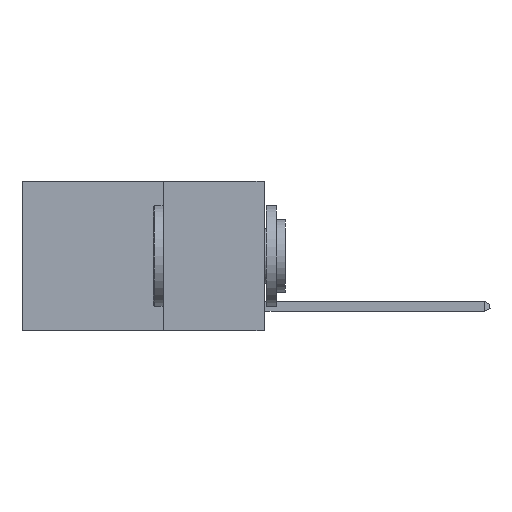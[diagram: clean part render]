
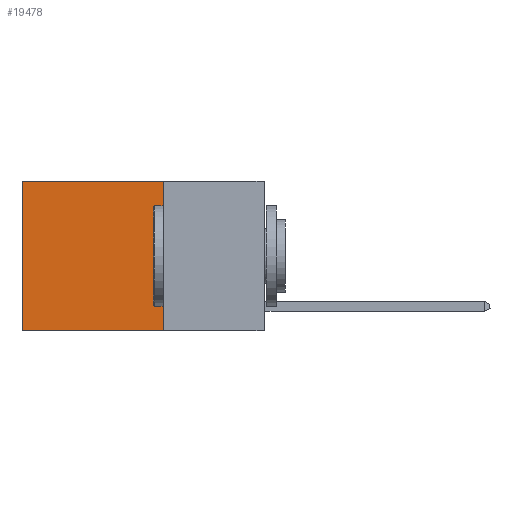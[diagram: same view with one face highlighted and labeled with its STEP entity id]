
A CAD part, left-side view. The second image highlights one B-rep face of the part: STEP entity #19478.
In plain terms, the highlighted planar face has unit normal (-1, 0, 0).
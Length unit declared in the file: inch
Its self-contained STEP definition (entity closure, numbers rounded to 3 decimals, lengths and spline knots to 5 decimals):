
#338 = CARTESIAN_POINT ( 'NONE',  ( 0.2625, 0.25, 0. ) ) ;
#354 = VECTOR ( 'NONE', #20214, 39.37008 ) ;
#499 = CARTESIAN_POINT ( 'NONE',  ( 0.2625, 0.25, 0. ) ) ;
#1576 = CARTESIAN_POINT ( 'NONE',  ( 0.2625, 0.25, -0.37 ) ) ;
#2954 = ORIENTED_EDGE ( 'NONE', *, *, #8389, .F. ) ;
#3614 = CARTESIAN_POINT ( 'NONE',  ( 0.2625, 0.6, 0. ) ) ;
#3741 = DIRECTION ( 'NONE',  ( 0., 0., -1. ) ) ;
#4375 = DIRECTION ( 'NONE',  ( 0., 0., -1. ) ) ;
#5207 = LINE ( 'NONE', #13923, #22955 ) ;
#5545 = CARTESIAN_POINT ( 'NONE',  ( 0.2625, 0.6, -0.37 ) ) ;
#5918 = FACE_OUTER_BOUND ( 'NONE', #6342, .T. ) ;
#6342 = EDGE_LOOP ( 'NONE', ( #15962, #17156, #2954, #9916 ) ) ;
#6417 = VECTOR ( 'NONE', #3741, 39.37008 ) ;
#7149 = LINE ( 'NONE', #338, #6417 ) ;
#7346 = VECTOR ( 'NONE', #10700, 39.37008 ) ;
#7847 = CARTESIAN_POINT ( 'NONE',  ( 0.2625, 0.6, 0. ) ) ;
#7977 = EDGE_CURVE ( 'NONE', #14332, #16102, #5207, .T. ) ;
#8014 = DIRECTION ( 'NONE',  ( 1., 0., 0. ) ) ;
#8389 = EDGE_CURVE ( 'NONE', #14332, #19967, #7149, .T. ) ;
#9604 = EDGE_CURVE ( 'NONE', #16102, #15600, #12453, .T. ) ;
#9916 = ORIENTED_EDGE ( 'NONE', *, *, #7977, .T. ) ;
#10388 = DIRECTION ( 'NONE',  ( 0., 1., 0. ) ) ;
#10700 = DIRECTION ( 'NONE',  ( 0., 0., -1. ) ) ;
#12453 = LINE ( 'NONE', #3614, #7346 ) ;
#13923 = CARTESIAN_POINT ( 'NONE',  ( 0.2625, 0.25, 0. ) ) ;
#14292 = AXIS2_PLACEMENT_3D ( 'NONE', #499, #8014, #4375 ) ;
#14332 = VERTEX_POINT ( 'NONE', #18263 ) ;
#15600 = VERTEX_POINT ( 'NONE', #5545 ) ;
#15962 = ORIENTED_EDGE ( 'NONE', *, *, #9604, .T. ) ;
#16102 = VERTEX_POINT ( 'NONE', #7847 ) ;
#16639 = PLANE ( 'NONE',  #14292 ) ;
#17156 = ORIENTED_EDGE ( 'NONE', *, *, #17828, .F. ) ;
#17742 = LINE ( 'NONE', #1576, #354 ) ;
#17828 = EDGE_CURVE ( 'NONE', #19967, #15600, #17742, .T. ) ;
#18263 = CARTESIAN_POINT ( 'NONE',  ( 0.2625, 0.25, 0. ) ) ;
#19478 = ADVANCED_FACE ( 'NONE', ( #5918 ), #16639, .F. ) ;
#19967 = VERTEX_POINT ( 'NONE', #20622 ) ;
#20214 = DIRECTION ( 'NONE',  ( 0., 1., 0. ) ) ;
#20622 = CARTESIAN_POINT ( 'NONE',  ( 0.2625, 0.25, -0.37 ) ) ;
#22955 = VECTOR ( 'NONE', #10388, 39.37008 ) ;
